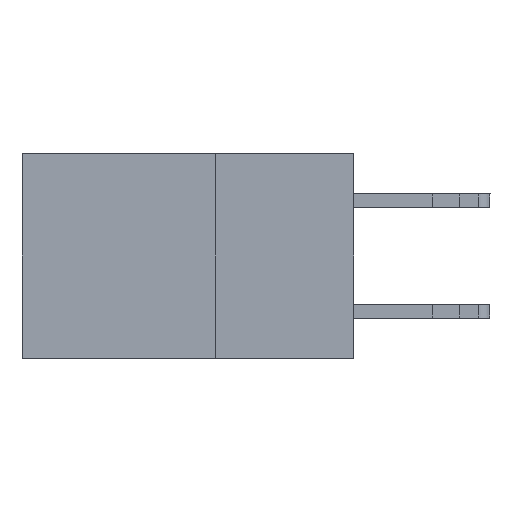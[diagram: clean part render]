
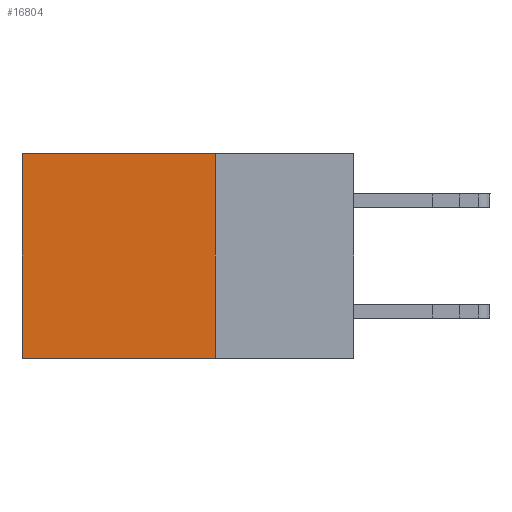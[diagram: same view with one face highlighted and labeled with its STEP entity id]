
A CAD part, left-side view. The second image highlights one B-rep face of the part: STEP entity #16804.
In plain terms, the highlighted planar face has unit normal (-1, 0, 0).
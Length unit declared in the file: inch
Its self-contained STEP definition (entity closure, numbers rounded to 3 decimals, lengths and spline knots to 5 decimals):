
#195 = EDGE_CURVE ( 'NONE', #8889, #13932, #7626, .T. ) ;
#766 = DIRECTION ( 'NONE',  ( 0., 0., -1. ) ) ;
#1014 = ORIENTED_EDGE ( 'NONE', *, *, #195, .F. ) ;
#1604 = CARTESIAN_POINT ( 'NONE',  ( 0.2875, 0.25, 0. ) ) ;
#1640 = EDGE_CURVE ( 'NONE', #5033, #4012, #18305, .T. ) ;
#2246 = ORIENTED_EDGE ( 'NONE', *, *, #5179, .T. ) ;
#2601 = CARTESIAN_POINT ( 'NONE',  ( 0.2875, 0.25, 0. ) ) ;
#3152 = DIRECTION ( 'NONE',  ( 0., 0., -1. ) ) ;
#3420 = LINE ( 'NONE', #13355, #3490 ) ;
#3490 = VECTOR ( 'NONE', #3152, 39.37008 ) ;
#3532 = CARTESIAN_POINT ( 'NONE',  ( 0.2875, 0.25, -0.37 ) ) ;
#4012 = VERTEX_POINT ( 'NONE', #17265 ) ;
#4249 = AXIS2_PLACEMENT_3D ( 'NONE', #17788, #9229, #766 ) ;
#4292 = EDGE_LOOP ( 'NONE', ( #2246, #1014, #4706, #7275 ) ) ;
#4574 = CARTESIAN_POINT ( 'NONE',  ( 0.2875, 0.25, 0. ) ) ;
#4706 = ORIENTED_EDGE ( 'NONE', *, *, #6826, .F. ) ;
#5033 = VERTEX_POINT ( 'NONE', #4574 ) ;
#5179 = EDGE_CURVE ( 'NONE', #4012, #13932, #3420, .T. ) ;
#6110 = VECTOR ( 'NONE', #7278, 39.37008 ) ;
#6324 = DIRECTION ( 'NONE',  ( 0., 1., 0. ) ) ;
#6826 = EDGE_CURVE ( 'NONE', #5033, #8889, #8677, .T. ) ;
#7275 = ORIENTED_EDGE ( 'NONE', *, *, #1640, .T. ) ;
#7278 = DIRECTION ( 'NONE',  ( 0., 0., -1. ) ) ;
#7626 = LINE ( 'NONE', #3532, #10671 ) ;
#7739 = CARTESIAN_POINT ( 'NONE',  ( 0.2875, 0.6, -0.37 ) ) ;
#7841 = FACE_OUTER_BOUND ( 'NONE', #4292, .T. ) ;
#8270 = DIRECTION ( 'NONE',  ( 0., 1., 0. ) ) ;
#8677 = LINE ( 'NONE', #1604, #6110 ) ;
#8889 = VERTEX_POINT ( 'NONE', #9654 ) ;
#9229 = DIRECTION ( 'NONE',  ( 1., 0., 0. ) ) ;
#9654 = CARTESIAN_POINT ( 'NONE',  ( 0.2875, 0.25, -0.37 ) ) ;
#10671 = VECTOR ( 'NONE', #6324, 39.37008 ) ;
#12102 = PLANE ( 'NONE',  #4249 ) ;
#13355 = CARTESIAN_POINT ( 'NONE',  ( 0.2875, 0.6, 0. ) ) ;
#13932 = VERTEX_POINT ( 'NONE', #7739 ) ;
#16715 = VECTOR ( 'NONE', #8270, 39.37008 ) ;
#16804 = ADVANCED_FACE ( 'NONE', ( #7841 ), #12102, .F. ) ;
#17265 = CARTESIAN_POINT ( 'NONE',  ( 0.2875, 0.6, 0. ) ) ;
#17788 = CARTESIAN_POINT ( 'NONE',  ( 0.2875, 0.25, 0. ) ) ;
#18305 = LINE ( 'NONE', #2601, #16715 ) ;
